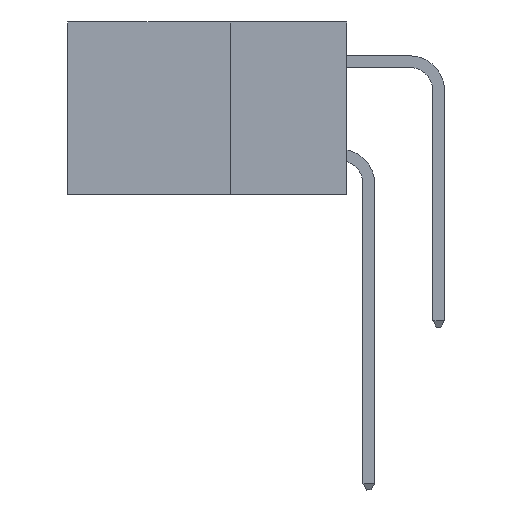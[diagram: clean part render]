
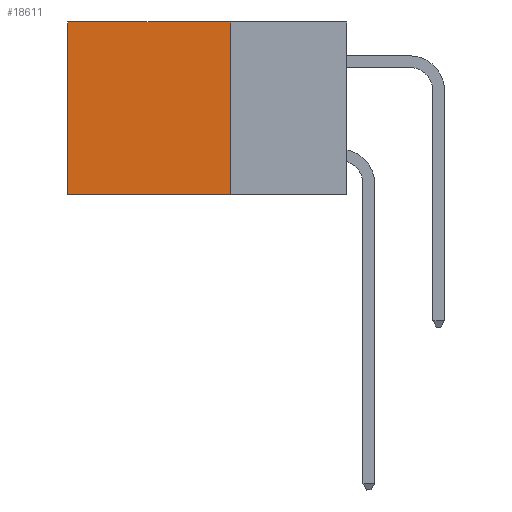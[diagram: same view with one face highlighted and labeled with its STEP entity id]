
A CAD part, left-side view. The second image highlights one B-rep face of the part: STEP entity #18611.
In plain terms, the highlighted planar face has unit normal (-1, 0, 0).
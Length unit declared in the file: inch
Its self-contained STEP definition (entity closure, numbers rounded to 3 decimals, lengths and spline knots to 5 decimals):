
#524 = VERTEX_POINT ( 'NONE', #16195 ) ;
#1728 = LINE ( 'NONE', #6040, #6235 ) ;
#2026 = DIRECTION ( 'NONE',  ( 0., 0., -1. ) ) ;
#2540 = VERTEX_POINT ( 'NONE', #3407 ) ;
#2751 = EDGE_CURVE ( 'NONE', #524, #10850, #1728, .T. ) ;
#2871 = AXIS2_PLACEMENT_3D ( 'NONE', #11235, #13992, #19220 ) ;
#3316 = ORIENTED_EDGE ( 'NONE', *, *, #11194, .F. ) ;
#3407 = CARTESIAN_POINT ( 'NONE',  ( 0.2875, 0.25, 0. ) ) ;
#3909 = CARTESIAN_POINT ( 'NONE',  ( 0.2875, 0.25, 0. ) ) ;
#4430 = LINE ( 'NONE', #3909, #6227 ) ;
#4682 = VECTOR ( 'NONE', #21303, 39.37008 ) ;
#6040 = CARTESIAN_POINT ( 'NONE',  ( 0.2875, 0.6, 0. ) ) ;
#6227 = VECTOR ( 'NONE', #9769, 39.37008 ) ;
#6235 = VECTOR ( 'NONE', #2026, 39.37008 ) ;
#8313 = LINE ( 'NONE', #19444, #4682 ) ;
#9769 = DIRECTION ( 'NONE',  ( 0., 1., 0. ) ) ;
#10242 = CARTESIAN_POINT ( 'NONE',  ( 0.2875, 0.25, 0. ) ) ;
#10372 = EDGE_LOOP ( 'NONE', ( #14534, #10489, #3316, #14549 ) ) ;
#10489 = ORIENTED_EDGE ( 'NONE', *, *, #13527, .F. ) ;
#10850 = VERTEX_POINT ( 'NONE', #19984 ) ;
#11194 = EDGE_CURVE ( 'NONE', #2540, #13881, #18303, .T. ) ;
#11235 = CARTESIAN_POINT ( 'NONE',  ( 0.2875, 0.25, 0. ) ) ;
#11631 = CARTESIAN_POINT ( 'NONE',  ( 0.2875, 0.25, -0.37 ) ) ;
#11955 = EDGE_CURVE ( 'NONE', #2540, #524, #4430, .T. ) ;
#12892 = VECTOR ( 'NONE', #23740, 39.37008 ) ;
#13527 = EDGE_CURVE ( 'NONE', #13881, #10850, #8313, .T. ) ;
#13881 = VERTEX_POINT ( 'NONE', #11631 ) ;
#13992 = DIRECTION ( 'NONE',  ( 1., 0., 0. ) ) ;
#14534 = ORIENTED_EDGE ( 'NONE', *, *, #2751, .T. ) ;
#14549 = ORIENTED_EDGE ( 'NONE', *, *, #11955, .T. ) ;
#16195 = CARTESIAN_POINT ( 'NONE',  ( 0.2875, 0.6, 0. ) ) ;
#17069 = FACE_OUTER_BOUND ( 'NONE', #10372, .T. ) ;
#18303 = LINE ( 'NONE', #10242, #12892 ) ;
#18611 = ADVANCED_FACE ( 'NONE', ( #17069 ), #22063, .F. ) ;
#19220 = DIRECTION ( 'NONE',  ( 0., 0., -1. ) ) ;
#19444 = CARTESIAN_POINT ( 'NONE',  ( 0.2875, 0.25, -0.37 ) ) ;
#19984 = CARTESIAN_POINT ( 'NONE',  ( 0.2875, 0.6, -0.37 ) ) ;
#21303 = DIRECTION ( 'NONE',  ( 0., 1., 0. ) ) ;
#22063 = PLANE ( 'NONE',  #2871 ) ;
#23740 = DIRECTION ( 'NONE',  ( 0., 0., -1. ) ) ;
